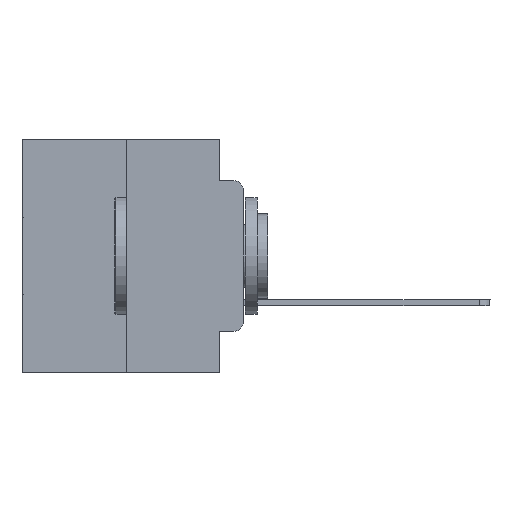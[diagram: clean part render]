
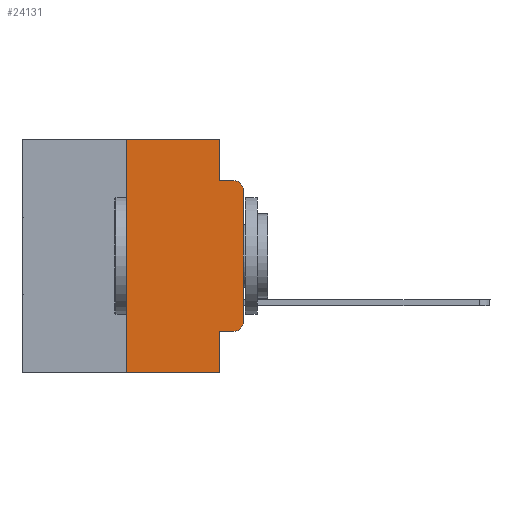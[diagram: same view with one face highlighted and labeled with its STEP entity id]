
A CAD part, left-side view. The second image highlights one B-rep face of the part: STEP entity #24131.
In plain terms, the highlighted planar face has unit normal (-1, 0, 0).
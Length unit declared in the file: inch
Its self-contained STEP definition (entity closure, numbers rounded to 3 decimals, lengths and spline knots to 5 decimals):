
#107 = DIRECTION ( 'NONE',  ( 0., -1., 0. ) ) ;
#153 = LINE ( 'NONE', #570, #15628 ) ;
#237 = DIRECTION ( 'NONE',  ( 0., -1., 0. ) ) ;
#570 = CARTESIAN_POINT ( 'NONE',  ( 0., 0.25, 0. ) ) ;
#672 = CARTESIAN_POINT ( 'NONE',  ( 0., 0.473, 0. ) ) ;
#1028 = CARTESIAN_POINT ( 'NONE',  ( 0., 0.051, 0. ) ) ;
#1066 = DIRECTION ( 'NONE',  ( 0., 0., -1. ) ) ;
#1161 = DIRECTION ( 'NONE',  ( -1., 0., 0. ) ) ;
#1304 = VERTEX_POINT ( 'NONE', #6198 ) ;
#1671 = VERTEX_POINT ( 'NONE', #13985 ) ;
#2500 = DIRECTION ( 'NONE',  ( 0., 0., -1. ) ) ;
#2501 = ORIENTED_EDGE ( 'NONE', *, *, #14606, .T. ) ;
#3161 = CARTESIAN_POINT ( 'NONE',  ( 0., 0.051, 0. ) ) ;
#3167 = EDGE_CURVE ( 'NONE', #7628, #13683, #15842, .T. ) ;
#4097 = VECTOR ( 'NONE', #107, 39.37008 ) ;
#4156 = CARTESIAN_POINT ( 'NONE',  ( 0., 0.25, 0. ) ) ;
#4432 = CARTESIAN_POINT ( 'NONE',  ( 0., 0.02, -0.4115 ) ) ;
#4718 = CARTESIAN_POINT ( 'NONE',  ( 0., 0., -0.1085 ) ) ;
#5190 = DIRECTION ( 'NONE',  ( 0., 0., 1. ) ) ;
#6198 = CARTESIAN_POINT ( 'NONE',  ( 0., 0.051, -0.5 ) ) ;
#6236 = VERTEX_POINT ( 'NONE', #4156 ) ;
#7178 = VECTOR ( 'NONE', #2500, 39.37008 ) ;
#7220 = VERTEX_POINT ( 'NONE', #11105 ) ;
#7379 = AXIS2_PLACEMENT_3D ( 'NONE', #672, #18644, #25336 ) ;
#7628 = VERTEX_POINT ( 'NONE', #3161 ) ;
#7705 = ORIENTED_EDGE ( 'NONE', *, *, #26493, .T. ) ;
#7859 = PLANE ( 'NONE',  #7379 ) ;
#7864 = LINE ( 'NONE', #10988, #10691 ) ;
#8344 = DIRECTION ( 'NONE',  ( 0., 0., -1. ) ) ;
#8370 = VECTOR ( 'NONE', #18872, 39.37008 ) ;
#8439 = VERTEX_POINT ( 'NONE', #4718 ) ;
#8615 = LINE ( 'NONE', #22670, #14866 ) ;
#8621 = EDGE_LOOP ( 'NONE', ( #2501, #7705, #15780, #28671, #23650, #19081, #21538, #16617, #11834, #20754 ) ) ;
#8708 = DIRECTION ( 'NONE',  ( 0., 0., -1. ) ) ;
#8821 = EDGE_CURVE ( 'NONE', #1671, #1304, #19859, .T. ) ;
#10580 = CIRCLE ( 'NONE', #25159, 0.02 ) ;
#10589 = FACE_OUTER_BOUND ( 'NONE', #8621, .T. ) ;
#10691 = VECTOR ( 'NONE', #18214, 39.37008 ) ;
#10854 = CARTESIAN_POINT ( 'NONE',  ( 0., 0.02, -0.1085 ) ) ;
#10988 = CARTESIAN_POINT ( 'NONE',  ( 0., 0.051, -0.0885 ) ) ;
#11105 = CARTESIAN_POINT ( 'NONE',  ( 0., 0., -0.3915 ) ) ;
#11196 = VERTEX_POINT ( 'NONE', #22762 ) ;
#11834 = ORIENTED_EDGE ( 'NONE', *, *, #17864, .T. ) ;
#13176 = VERTEX_POINT ( 'NONE', #4432 ) ;
#13268 = CARTESIAN_POINT ( 'NONE',  ( 0., 0.051, -0.0885 ) ) ;
#13272 = LINE ( 'NONE', #22636, #4097 ) ;
#13277 = AXIS2_PLACEMENT_3D ( 'NONE', #10854, #28386, #8708 ) ;
#13303 = CARTESIAN_POINT ( 'NONE',  ( 0., 0.02, -0.0885 ) ) ;
#13400 = EDGE_CURVE ( 'NONE', #13176, #7220, #10580, .T. ) ;
#13683 = VERTEX_POINT ( 'NONE', #13268 ) ;
#13985 = CARTESIAN_POINT ( 'NONE',  ( 0., 0.25, -0.5 ) ) ;
#14541 = CARTESIAN_POINT ( 'NONE',  ( 0., 0.02, -0.3915 ) ) ;
#14606 = EDGE_CURVE ( 'NONE', #7220, #8439, #18203, .T. ) ;
#14866 = VECTOR ( 'NONE', #237, 39.37008 ) ;
#15628 = VECTOR ( 'NONE', #5190, 39.37008 ) ;
#15780 = ORIENTED_EDGE ( 'NONE', *, *, #16812, .F. ) ;
#15842 = LINE ( 'NONE', #1028, #21372 ) ;
#16617 = ORIENTED_EDGE ( 'NONE', *, *, #16907, .F. ) ;
#16812 = EDGE_CURVE ( 'NONE', #13683, #20571, #7864, .T. ) ;
#16868 = CARTESIAN_POINT ( 'NONE',  ( 0., 0.473, -0.5 ) ) ;
#16907 = EDGE_CURVE ( 'NONE', #11196, #1304, #19806, .T. ) ;
#16914 = CARTESIAN_POINT ( 'NONE',  ( 0., 0., 0. ) ) ;
#17864 = EDGE_CURVE ( 'NONE', #11196, #13176, #8615, .T. ) ;
#18203 = LINE ( 'NONE', #16914, #8370 ) ;
#18214 = DIRECTION ( 'NONE',  ( 0., -1., 0. ) ) ;
#18376 = EDGE_CURVE ( 'NONE', #6236, #7628, #13272, .T. ) ;
#18644 = DIRECTION ( 'NONE',  ( 1., 0., 0. ) ) ;
#18872 = DIRECTION ( 'NONE',  ( 0., 0., 1. ) ) ;
#19081 = ORIENTED_EDGE ( 'NONE', *, *, #27420, .F. ) ;
#19126 = DIRECTION ( 'NONE',  ( 0., -1., 0. ) ) ;
#19806 = LINE ( 'NONE', #27067, #7178 ) ;
#19859 = LINE ( 'NONE', #16868, #21582 ) ;
#20571 = VERTEX_POINT ( 'NONE', #13303 ) ;
#20754 = ORIENTED_EDGE ( 'NONE', *, *, #13400, .T. ) ;
#21372 = VECTOR ( 'NONE', #8344, 39.37008 ) ;
#21538 = ORIENTED_EDGE ( 'NONE', *, *, #8821, .T. ) ;
#21582 = VECTOR ( 'NONE', #19126, 39.37008 ) ;
#22636 = CARTESIAN_POINT ( 'NONE',  ( 0., 0.473, 0. ) ) ;
#22670 = CARTESIAN_POINT ( 'NONE',  ( 0., 0.051, -0.4115 ) ) ;
#22762 = CARTESIAN_POINT ( 'NONE',  ( 0., 0.051, -0.4115 ) ) ;
#23650 = ORIENTED_EDGE ( 'NONE', *, *, #18376, .F. ) ;
#24131 = ADVANCED_FACE ( 'NONE', ( #10589 ), #7859, .F. ) ;
#25159 = AXIS2_PLACEMENT_3D ( 'NONE', #14541, #1161, #1066 ) ;
#25336 = DIRECTION ( 'NONE',  ( 0., 0., -1. ) ) ;
#26493 = EDGE_CURVE ( 'NONE', #8439, #20571, #28186, .T. ) ;
#27067 = CARTESIAN_POINT ( 'NONE',  ( 0., 0.051, 0. ) ) ;
#27420 = EDGE_CURVE ( 'NONE', #1671, #6236, #153, .T. ) ;
#28186 = CIRCLE ( 'NONE', #13277, 0.02 ) ;
#28386 = DIRECTION ( 'NONE',  ( -1., 0., 0. ) ) ;
#28671 = ORIENTED_EDGE ( 'NONE', *, *, #3167, .F. ) ;
